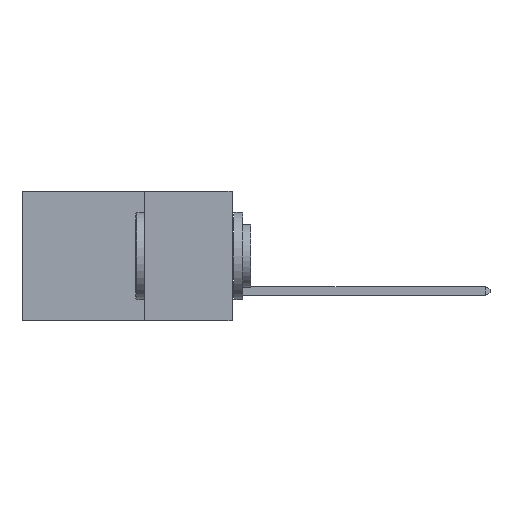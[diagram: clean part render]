
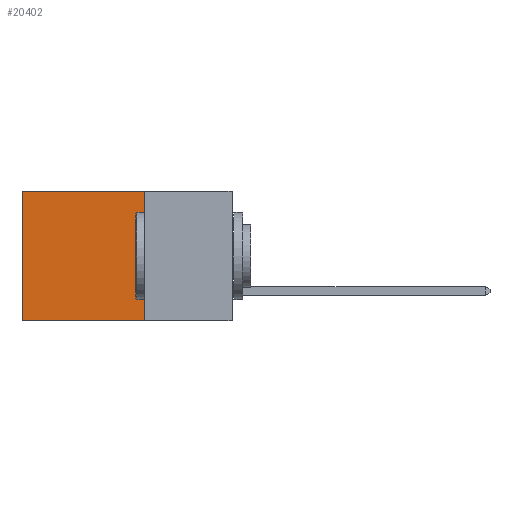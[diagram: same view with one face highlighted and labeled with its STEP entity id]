
A CAD part, left-side view. The second image highlights one B-rep face of the part: STEP entity #20402.
In plain terms, the highlighted planar face has unit normal (-1, 0, 0).
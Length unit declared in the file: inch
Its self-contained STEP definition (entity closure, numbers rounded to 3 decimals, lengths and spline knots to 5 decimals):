
#293 = CARTESIAN_POINT ( 'NONE',  ( 0.2875, 0.25, -0.37 ) ) ;
#850 = VERTEX_POINT ( 'NONE', #5889 ) ;
#1671 = LINE ( 'NONE', #21403, #7034 ) ;
#3048 = EDGE_CURVE ( 'NONE', #850, #19899, #26006, .T. ) ;
#5601 = CARTESIAN_POINT ( 'NONE',  ( 0.2875, 0.25, 0. ) ) ;
#5889 = CARTESIAN_POINT ( 'NONE',  ( 0.2875, 0.25, -0.37 ) ) ;
#6195 = CARTESIAN_POINT ( 'NONE',  ( 0.2875, 0.25, 0. ) ) ;
#7034 = VECTOR ( 'NONE', #23707, 39.37008 ) ;
#7835 = VECTOR ( 'NONE', #18551, 39.37008 ) ;
#8464 = VECTOR ( 'NONE', #19853, 39.37008 ) ;
#8830 = DIRECTION ( 'NONE',  ( 1., 0., 0. ) ) ;
#9367 = EDGE_CURVE ( 'NONE', #21169, #850, #20554, .T. ) ;
#10202 = DIRECTION ( 'NONE',  ( 0., 1., 0. ) ) ;
#10762 = ORIENTED_EDGE ( 'NONE', *, *, #18978, .T. ) ;
#10908 = FACE_OUTER_BOUND ( 'NONE', #21901, .T. ) ;
#11569 = AXIS2_PLACEMENT_3D ( 'NONE', #22445, #8830, #24737 ) ;
#13402 = CARTESIAN_POINT ( 'NONE',  ( 0.2875, 0.6, -0.37 ) ) ;
#14020 = VECTOR ( 'NONE', #10202, 39.37008 ) ;
#14508 = ORIENTED_EDGE ( 'NONE', *, *, #25889, .T. ) ;
#14651 = ORIENTED_EDGE ( 'NONE', *, *, #9367, .F. ) ;
#18551 = DIRECTION ( 'NONE',  ( 0., 1., 0. ) ) ;
#18978 = EDGE_CURVE ( 'NONE', #28312, #19899, #1671, .T. ) ;
#19853 = DIRECTION ( 'NONE',  ( 0., 0., -1. ) ) ;
#19899 = VERTEX_POINT ( 'NONE', #13402 ) ;
#20094 = LINE ( 'NONE', #5601, #14020 ) ;
#20402 = ADVANCED_FACE ( 'NONE', ( #10908 ), #26938, .F. ) ;
#20554 = LINE ( 'NONE', #6195, #8464 ) ;
#21169 = VERTEX_POINT ( 'NONE', #25135 ) ;
#21403 = CARTESIAN_POINT ( 'NONE',  ( 0.2875, 0.6, 0. ) ) ;
#21901 = EDGE_LOOP ( 'NONE', ( #10762, #26128, #14651, #14508 ) ) ;
#22445 = CARTESIAN_POINT ( 'NONE',  ( 0.2875, 0.25, 0. ) ) ;
#23363 = CARTESIAN_POINT ( 'NONE',  ( 0.2875, 0.6, 0. ) ) ;
#23707 = DIRECTION ( 'NONE',  ( 0., 0., -1. ) ) ;
#24737 = DIRECTION ( 'NONE',  ( 0., 0., -1. ) ) ;
#25135 = CARTESIAN_POINT ( 'NONE',  ( 0.2875, 0.25, 0. ) ) ;
#25889 = EDGE_CURVE ( 'NONE', #21169, #28312, #20094, .T. ) ;
#26006 = LINE ( 'NONE', #293, #7835 ) ;
#26128 = ORIENTED_EDGE ( 'NONE', *, *, #3048, .F. ) ;
#26938 = PLANE ( 'NONE',  #11569 ) ;
#28312 = VERTEX_POINT ( 'NONE', #23363 ) ;
